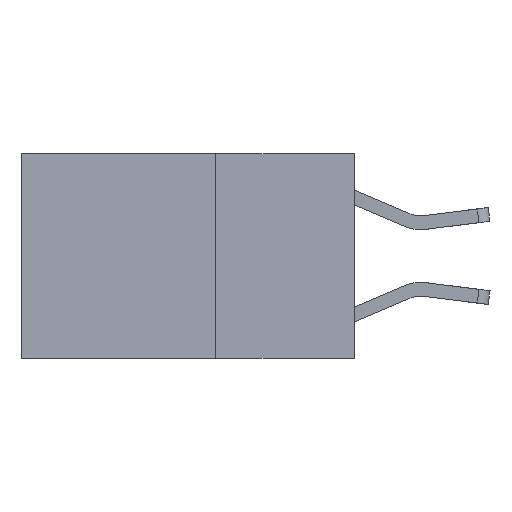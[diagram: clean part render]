
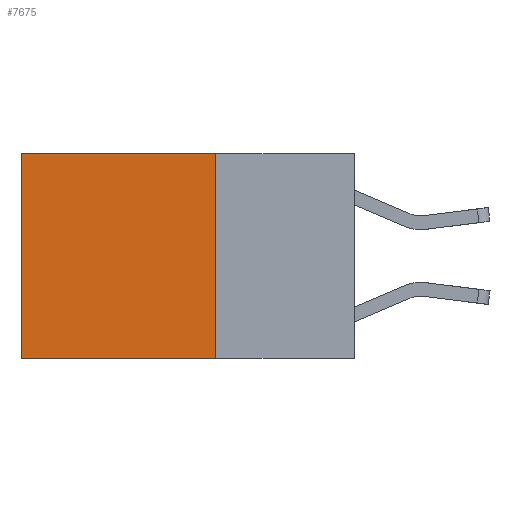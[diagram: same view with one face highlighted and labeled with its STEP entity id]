
A CAD part, left-side view. The second image highlights one B-rep face of the part: STEP entity #7675.
In plain terms, the highlighted planar face has unit normal (-1, 0, 0).
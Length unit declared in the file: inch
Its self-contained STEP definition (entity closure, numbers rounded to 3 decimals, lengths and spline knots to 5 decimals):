
#45 = EDGE_CURVE ( 'NONE', #5693, #989, #233, .T. ) ;
#183 = EDGE_LOOP ( 'NONE', ( #6052, #3989, #1416, #11182 ) ) ;
#233 = LINE ( 'NONE', #2283, #9942 ) ;
#559 = PLANE ( 'NONE',  #686 ) ;
#662 = CARTESIAN_POINT ( 'NONE',  ( 0.2625, 0.25, 0. ) ) ;
#686 = AXIS2_PLACEMENT_3D ( 'NONE', #3494, #10210, #4439 ) ;
#989 = VERTEX_POINT ( 'NONE', #1901 ) ;
#1416 = ORIENTED_EDGE ( 'NONE', *, *, #3787, .F. ) ;
#1901 = CARTESIAN_POINT ( 'NONE',  ( 0.2625, 0.6, -0.37 ) ) ;
#2121 = CARTESIAN_POINT ( 'NONE',  ( 0.2625, 0.25, 0. ) ) ;
#2248 = CARTESIAN_POINT ( 'NONE',  ( 0.2625, 0.25, 0. ) ) ;
#2283 = CARTESIAN_POINT ( 'NONE',  ( 0.2625, 0.6, 0. ) ) ;
#2787 = VERTEX_POINT ( 'NONE', #662 ) ;
#3494 = CARTESIAN_POINT ( 'NONE',  ( 0.2625, 0.25, 0. ) ) ;
#3787 = EDGE_CURVE ( 'NONE', #2787, #7497, #7912, .T. ) ;
#3989 = ORIENTED_EDGE ( 'NONE', *, *, #10581, .F. ) ;
#4439 = DIRECTION ( 'NONE',  ( 0., 0., -1. ) ) ;
#5693 = VERTEX_POINT ( 'NONE', #11598 ) ;
#6052 = ORIENTED_EDGE ( 'NONE', *, *, #45, .T. ) ;
#6190 = CARTESIAN_POINT ( 'NONE',  ( 0.2625, 0.25, -0.37 ) ) ;
#6468 = CARTESIAN_POINT ( 'NONE',  ( 0.2625, 0.25, -0.37 ) ) ;
#7104 = VECTOR ( 'NONE', #10648, 39.37008 ) ;
#7143 = DIRECTION ( 'NONE',  ( 0., 0., -1. ) ) ;
#7479 = DIRECTION ( 'NONE',  ( 0., 1., 0. ) ) ;
#7497 = VERTEX_POINT ( 'NONE', #6190 ) ;
#7512 = VECTOR ( 'NONE', #7479, 39.37008 ) ;
#7607 = VECTOR ( 'NONE', #9934, 39.37008 ) ;
#7675 = ADVANCED_FACE ( 'NONE', ( #12045 ), #559, .F. ) ;
#7821 = LINE ( 'NONE', #6468, #7512 ) ;
#7912 = LINE ( 'NONE', #2248, #7607 ) ;
#8712 = EDGE_CURVE ( 'NONE', #2787, #5693, #9624, .T. ) ;
#9624 = LINE ( 'NONE', #2121, #7104 ) ;
#9934 = DIRECTION ( 'NONE',  ( 0., 0., -1. ) ) ;
#9942 = VECTOR ( 'NONE', #7143, 39.37008 ) ;
#10210 = DIRECTION ( 'NONE',  ( 1., 0., 0. ) ) ;
#10581 = EDGE_CURVE ( 'NONE', #7497, #989, #7821, .T. ) ;
#10648 = DIRECTION ( 'NONE',  ( 0., 1., 0. ) ) ;
#11182 = ORIENTED_EDGE ( 'NONE', *, *, #8712, .T. ) ;
#11598 = CARTESIAN_POINT ( 'NONE',  ( 0.2625, 0.6, 0. ) ) ;
#12045 = FACE_OUTER_BOUND ( 'NONE', #183, .T. ) ;
